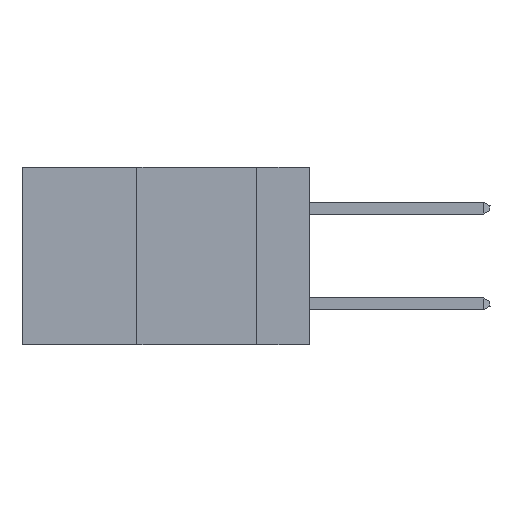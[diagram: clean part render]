
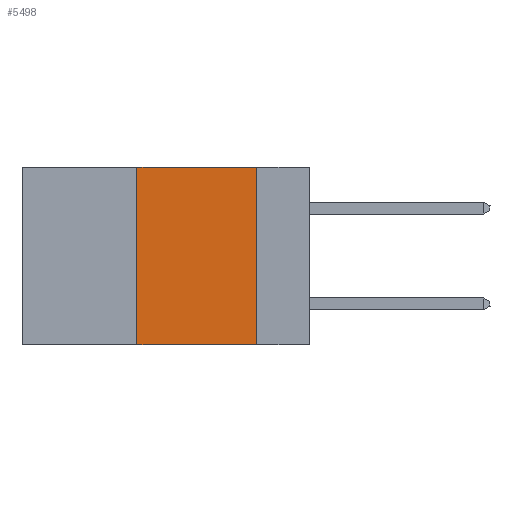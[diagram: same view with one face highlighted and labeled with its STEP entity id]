
A CAD part, left-side view. The second image highlights one B-rep face of the part: STEP entity #5498.
In plain terms, the highlighted planar face has unit normal (-1, 0, 0).
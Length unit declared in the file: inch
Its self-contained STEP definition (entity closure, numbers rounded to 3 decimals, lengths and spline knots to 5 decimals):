
#426 = ORIENTED_EDGE ( 'NONE', *, *, #9246, .T. ) ;
#1296 = EDGE_CURVE ( 'NONE', #3911, #21618, #14126, .T. ) ;
#2023 = CARTESIAN_POINT ( 'NONE',  ( 0., 0.36, 0. ) ) ;
#2313 = EDGE_CURVE ( 'NONE', #13602, #21230, #10422, .T. ) ;
#2689 = LINE ( 'NONE', #13257, #7340 ) ;
#3076 = VECTOR ( 'NONE', #21535, 39.37008 ) ;
#3911 = VERTEX_POINT ( 'NONE', #14783 ) ;
#4810 = AXIS2_PLACEMENT_3D ( 'NONE', #13667, #12080, #11851 ) ;
#5498 = ADVANCED_FACE ( 'NONE', ( #24667 ), #18447, .F. ) ;
#6526 = EDGE_CURVE ( 'NONE', #21230, #3911, #2689, .T. ) ;
#7340 = VECTOR ( 'NONE', #11020, 39.37008 ) ;
#8424 = LINE ( 'NONE', #20794, #19925 ) ;
#9118 = CARTESIAN_POINT ( 'NONE',  ( 0., 0.36, -0.37 ) ) ;
#9246 = EDGE_CURVE ( 'NONE', #13602, #21618, #8424, .T. ) ;
#10422 = LINE ( 'NONE', #2023, #20711 ) ;
#11020 = DIRECTION ( 'NONE',  ( 0., -1., 0. ) ) ;
#11851 = DIRECTION ( 'NONE',  ( 0., 0., -1. ) ) ;
#12080 = DIRECTION ( 'NONE',  ( 1., 0., 0. ) ) ;
#13257 = CARTESIAN_POINT ( 'NONE',  ( 0., 0.6, 0. ) ) ;
#13284 = ORIENTED_EDGE ( 'NONE', *, *, #1296, .F. ) ;
#13602 = VERTEX_POINT ( 'NONE', #9118 ) ;
#13667 = CARTESIAN_POINT ( 'NONE',  ( 0., 0.6, 0. ) ) ;
#14126 = LINE ( 'NONE', #23759, #3076 ) ;
#14783 = CARTESIAN_POINT ( 'NONE',  ( 0., 0.11, 0. ) ) ;
#16954 = DIRECTION ( 'NONE',  ( 0., -1., 0. ) ) ;
#17758 = DIRECTION ( 'NONE',  ( 0., 0., 1. ) ) ;
#18447 = PLANE ( 'NONE',  #4810 ) ;
#19010 = EDGE_LOOP ( 'NONE', ( #13284, #25274, #19511, #426 ) ) ;
#19511 = ORIENTED_EDGE ( 'NONE', *, *, #2313, .F. ) ;
#19925 = VECTOR ( 'NONE', #16954, 39.37008 ) ;
#20016 = CARTESIAN_POINT ( 'NONE',  ( 0., 0.11, -0.37 ) ) ;
#20711 = VECTOR ( 'NONE', #17758, 39.37008 ) ;
#20794 = CARTESIAN_POINT ( 'NONE',  ( 0., 0.6, -0.37 ) ) ;
#21230 = VERTEX_POINT ( 'NONE', #24696 ) ;
#21535 = DIRECTION ( 'NONE',  ( 0., 0., -1. ) ) ;
#21618 = VERTEX_POINT ( 'NONE', #20016 ) ;
#23759 = CARTESIAN_POINT ( 'NONE',  ( 0., 0.11, 0. ) ) ;
#24667 = FACE_OUTER_BOUND ( 'NONE', #19010, .T. ) ;
#24696 = CARTESIAN_POINT ( 'NONE',  ( 0., 0.36, 0. ) ) ;
#25274 = ORIENTED_EDGE ( 'NONE', *, *, #6526, .F. ) ;
